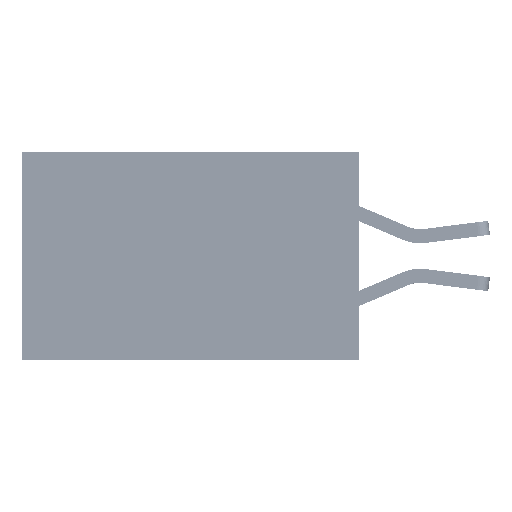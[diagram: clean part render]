
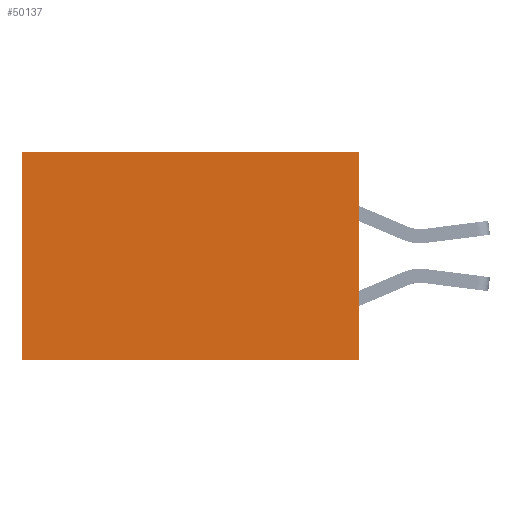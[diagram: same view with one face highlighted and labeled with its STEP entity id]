
A CAD part, left-side view. The second image highlights one B-rep face of the part: STEP entity #50137.
In plain terms, the highlighted planar face has unit normal (-1, 0, 0).
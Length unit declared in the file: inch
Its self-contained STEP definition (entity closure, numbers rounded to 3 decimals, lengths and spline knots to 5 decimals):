
#311 = ORIENTED_EDGE ( 'NONE', *, *, #38482, .T. ) ;
#950 = CARTESIAN_POINT ( 'NONE',  ( 0.2875, 0., 0. ) ) ;
#2236 = CARTESIAN_POINT ( 'NONE',  ( 0.2875, 0., 0. ) ) ;
#3300 = CARTESIAN_POINT ( 'NONE',  ( 0.2875, 0., -0.37 ) ) ;
#3662 = CARTESIAN_POINT ( 'NONE',  ( 0.2875, 0.6, 0. ) ) ;
#5666 = VERTEX_POINT ( 'NONE', #6733 ) ;
#6733 = CARTESIAN_POINT ( 'NONE',  ( 0.2875, 0., 0. ) ) ;
#6838 = ORIENTED_EDGE ( 'NONE', *, *, #50911, .F. ) ;
#8149 = DIRECTION ( 'NONE',  ( 0., 0., -1. ) ) ;
#9357 = LINE ( 'NONE', #3662, #42248 ) ;
#10695 = CARTESIAN_POINT ( 'NONE',  ( 0.2875, 0.6, -0.37 ) ) ;
#11307 = VECTOR ( 'NONE', #35842, 39.37008 ) ;
#14617 = DIRECTION ( 'NONE',  ( 0., 1., 0. ) ) ;
#15257 = AXIS2_PLACEMENT_3D ( 'NONE', #2236, #50337, #35404 ) ;
#19436 = EDGE_CURVE ( 'NONE', #5666, #22604, #20990, .T. ) ;
#20561 = EDGE_CURVE ( 'NONE', #5666, #46709, #29577, .T. ) ;
#20990 = LINE ( 'NONE', #950, #31508 ) ;
#22604 = VERTEX_POINT ( 'NONE', #3300 ) ;
#24998 = ORIENTED_EDGE ( 'NONE', *, *, #19436, .F. ) ;
#27852 = EDGE_LOOP ( 'NONE', ( #311, #6838, #24998, #30213 ) ) ;
#29577 = LINE ( 'NONE', #42184, #49396 ) ;
#29887 = LINE ( 'NONE', #43949, #11307 ) ;
#30213 = ORIENTED_EDGE ( 'NONE', *, *, #20561, .T. ) ;
#31508 = VECTOR ( 'NONE', #8149, 39.37008 ) ;
#31921 = CARTESIAN_POINT ( 'NONE',  ( 0.2875, 0.6, 0. ) ) ;
#35404 = DIRECTION ( 'NONE',  ( 0., 0., -1. ) ) ;
#35842 = DIRECTION ( 'NONE',  ( 0., 1., 0. ) ) ;
#38204 = FACE_OUTER_BOUND ( 'NONE', #27852, .T. ) ;
#38482 = EDGE_CURVE ( 'NONE', #46709, #45873, #9357, .T. ) ;
#42184 = CARTESIAN_POINT ( 'NONE',  ( 0.2875, 0., 0. ) ) ;
#42248 = VECTOR ( 'NONE', #44471, 39.37008 ) ;
#43949 = CARTESIAN_POINT ( 'NONE',  ( 0.2875, 0., -0.37 ) ) ;
#44471 = DIRECTION ( 'NONE',  ( 0., 0., -1. ) ) ;
#45873 = VERTEX_POINT ( 'NONE', #10695 ) ;
#46709 = VERTEX_POINT ( 'NONE', #31921 ) ;
#49396 = VECTOR ( 'NONE', #14617, 39.37008 ) ;
#50137 = ADVANCED_FACE ( 'NONE', ( #38204 ), #50168, .F. ) ;
#50168 = PLANE ( 'NONE',  #15257 ) ;
#50337 = DIRECTION ( 'NONE',  ( 1., 0., 0. ) ) ;
#50911 = EDGE_CURVE ( 'NONE', #22604, #45873, #29887, .T. ) ;
